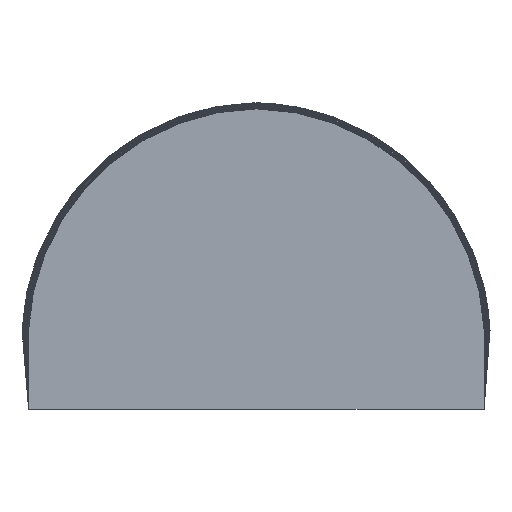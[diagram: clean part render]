
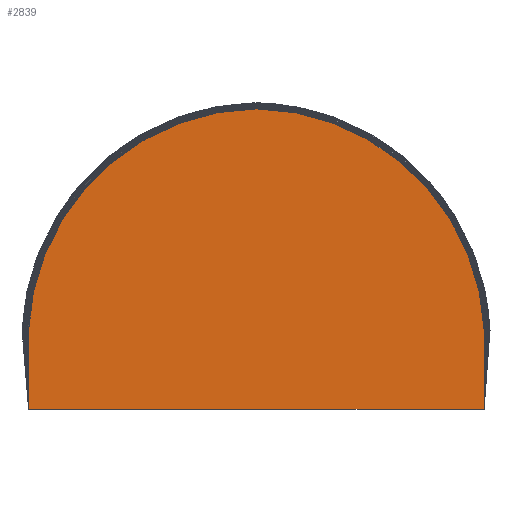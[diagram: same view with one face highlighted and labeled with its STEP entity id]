
A CAD part, front view. The second image highlights one B-rep face of the part: STEP entity #2839.
In plain terms, the highlighted planar face has unit normal (0, -1, 0).
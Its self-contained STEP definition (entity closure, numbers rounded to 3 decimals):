
#139=CIRCLE('',#3070,6.705);
#141=CIRCLE('',#3073,6.705);
#268=FACE_OUTER_BOUND('',#426,.T.);
#426=EDGE_LOOP('',(#2123,#2124,#2125,#2126,#2127));
#563=LINE('',#4029,#786);
#649=LINE('',#4787,#872);
#650=LINE('',#4790,#873);
#786=VECTOR('',#3290,10.);
#872=VECTOR('',#3516,10.);
#873=VECTOR('',#3519,10.);
#1148=VERTEX_POINT('',#4026);
#1149=VERTEX_POINT('',#4028);
#1252=VERTEX_POINT('',#4785);
#1253=VERTEX_POINT('',#4789);
#1256=VERTEX_POINT('',#4797);
#1440=EDGE_CURVE('',#1149,#1148,#563,.T.);
#1584=EDGE_CURVE('',#1148,#1252,#649,.T.);
#1585=EDGE_CURVE('',#1253,#1149,#650,.T.);
#1589=EDGE_CURVE('',#1256,#1253,#139,.T.);
#1592=EDGE_CURVE('',#1252,#1256,#141,.T.);
#2123=ORIENTED_EDGE('',*,*,#1440,.T.);
#2124=ORIENTED_EDGE('',*,*,#1584,.T.);
#2125=ORIENTED_EDGE('',*,*,#1592,.T.);
#2126=ORIENTED_EDGE('',*,*,#1589,.T.);
#2127=ORIENTED_EDGE('',*,*,#1585,.T.);
#2762=PLANE('',#3074);
#2839=ADVANCED_FACE('',(#268),#2762,.F.);
#3070=AXIS2_PLACEMENT_3D('',#4798,#3526,#3527);
#3073=AXIS2_PLACEMENT_3D('',#4802,#3533,#3534);
#3074=AXIS2_PLACEMENT_3D('',#4803,#3535,#3536);
#3290=DIRECTION('',(1.,0.,0.));
#3516=DIRECTION('',(0.,0.,1.));
#3519=DIRECTION('',(0.,0.,-1.));
#3526=DIRECTION('center_axis',(0.,-1.,0.));
#3527=DIRECTION('ref_axis',(-0.999,0.,0.046));
#3533=DIRECTION('center_axis',(0.,-1.,0.));
#3534=DIRECTION('ref_axis',(0.017,0.,1.));
#3535=DIRECTION('center_axis',(0.,1.,0.));
#3536=DIRECTION('ref_axis',(0.,0.,1.));
#4026=CARTESIAN_POINT('',(-6.092,-239.95,-29.838));
#4028=CARTESIAN_POINT('',(-19.261,-239.951,-29.838));
#4029=CARTESIAN_POINT('',(-0.692,-239.95,-29.838));
#4785=CARTESIAN_POINT('',(-6.092,-239.95,-27.55));
#4787=CARTESIAN_POINT('',(-6.092,-239.95,-52.126));
#4789=CARTESIAN_POINT('',(-19.261,-239.951,-27.55));
#4790=CARTESIAN_POINT('',(-19.261,-239.951,-27.55));
#4797=CARTESIAN_POINT('',(-12.677,-239.95,-21.152));
#4798=CARTESIAN_POINT('Origin',(-12.563,-239.95,-27.856));
#4802=CARTESIAN_POINT('Origin',(-12.79,-239.95,-27.856));
#4803=CARTESIAN_POINT('Origin',(-12.677,-239.95,-39.838));
